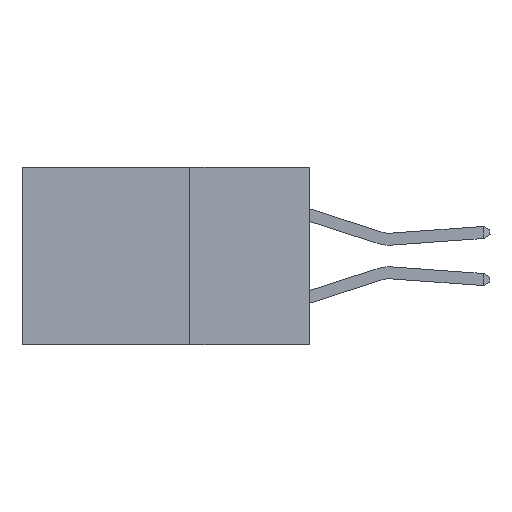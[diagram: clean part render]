
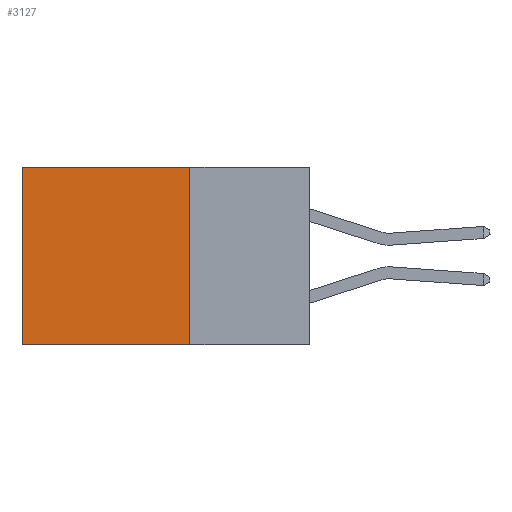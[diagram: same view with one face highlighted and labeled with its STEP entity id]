
A CAD part, left-side view. The second image highlights one B-rep face of the part: STEP entity #3127.
In plain terms, the highlighted planar face has unit normal (-1, 0, 0).
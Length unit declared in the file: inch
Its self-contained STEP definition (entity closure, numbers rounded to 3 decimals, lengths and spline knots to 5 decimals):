
#1019 = EDGE_CURVE ( 'NONE', #10616, #12043, #3787, .T. ) ;
#1048 = VERTEX_POINT ( 'NONE', #7557 ) ;
#2822 = CARTESIAN_POINT ( 'NONE',  ( 0.2615, 0.25, 0. ) ) ;
#3096 = LINE ( 'NONE', #10639, #9407 ) ;
#3127 = ADVANCED_FACE ( 'NONE', ( #4003 ), #7050, .F. ) ;
#3406 = LINE ( 'NONE', #6589, #6444 ) ;
#3471 = CARTESIAN_POINT ( 'NONE',  ( 0.2615, 0.6, 0. ) ) ;
#3787 = LINE ( 'NONE', #2822, #6430 ) ;
#4001 = AXIS2_PLACEMENT_3D ( 'NONE', #6394, #14492, #14454 ) ;
#4003 = FACE_OUTER_BOUND ( 'NONE', #14535, .T. ) ;
#4060 = VERTEX_POINT ( 'NONE', #10131 ) ;
#5370 = ORIENTED_EDGE ( 'NONE', *, *, #1019, .T. ) ;
#6344 = EDGE_CURVE ( 'NONE', #1048, #4060, #8285, .T. ) ;
#6394 = CARTESIAN_POINT ( 'NONE',  ( 0.2615, 0.25, -0.37 ) ) ;
#6430 = VECTOR ( 'NONE', #12425, 39.37008 ) ;
#6444 = VECTOR ( 'NONE', #6625, 39.37008 ) ;
#6589 = CARTESIAN_POINT ( 'NONE',  ( 0.2615, 0.6, -0.37 ) ) ;
#6625 = DIRECTION ( 'NONE',  ( 0., 0., -1. ) ) ;
#7050 = PLANE ( 'NONE',  #4001 ) ;
#7120 = EDGE_CURVE ( 'NONE', #10616, #1048, #3096, .T. ) ;
#7557 = CARTESIAN_POINT ( 'NONE',  ( 0.2615, 0.25, -0.37 ) ) ;
#8285 = LINE ( 'NONE', #14269, #11151 ) ;
#9407 = VECTOR ( 'NONE', #10958, 39.37008 ) ;
#10131 = CARTESIAN_POINT ( 'NONE',  ( 0.2615, 0.6, -0.37 ) ) ;
#10616 = VERTEX_POINT ( 'NONE', #13793 ) ;
#10639 = CARTESIAN_POINT ( 'NONE',  ( 0.2615, 0.25, -0.37 ) ) ;
#10958 = DIRECTION ( 'NONE',  ( 0., 0., -1. ) ) ;
#11090 = ORIENTED_EDGE ( 'NONE', *, *, #7120, .F. ) ;
#11151 = VECTOR ( 'NONE', #14634, 39.37008 ) ;
#11672 = EDGE_CURVE ( 'NONE', #12043, #4060, #3406, .T. ) ;
#12043 = VERTEX_POINT ( 'NONE', #3471 ) ;
#12425 = DIRECTION ( 'NONE',  ( 0., 1., 0. ) ) ;
#12634 = ORIENTED_EDGE ( 'NONE', *, *, #11672, .T. ) ;
#13793 = CARTESIAN_POINT ( 'NONE',  ( 0.2615, 0.25, 0. ) ) ;
#14269 = CARTESIAN_POINT ( 'NONE',  ( 0.2615, 0.25, -0.37 ) ) ;
#14454 = DIRECTION ( 'NONE',  ( 0., 0., -1. ) ) ;
#14492 = DIRECTION ( 'NONE',  ( 1., 0., 0. ) ) ;
#14535 = EDGE_LOOP ( 'NONE', ( #12634, #15236, #11090, #5370 ) ) ;
#14634 = DIRECTION ( 'NONE',  ( 0., 1., 0. ) ) ;
#15236 = ORIENTED_EDGE ( 'NONE', *, *, #6344, .F. ) ;
